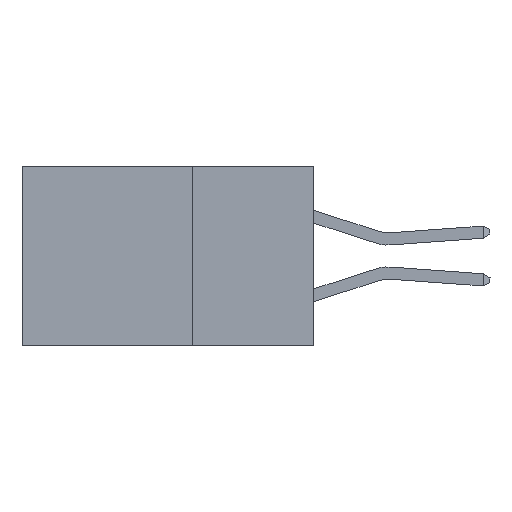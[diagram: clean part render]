
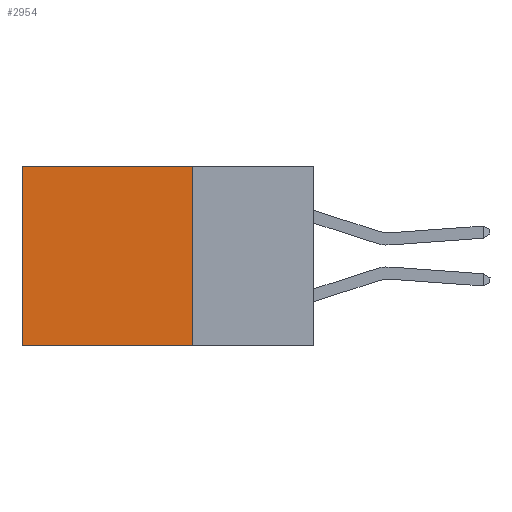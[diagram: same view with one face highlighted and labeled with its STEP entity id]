
A CAD part, left-side view. The second image highlights one B-rep face of the part: STEP entity #2954.
In plain terms, the highlighted planar face has unit normal (-1, 0, 0).
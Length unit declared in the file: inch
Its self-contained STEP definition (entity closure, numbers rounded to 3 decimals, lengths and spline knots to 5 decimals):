
#363 = CARTESIAN_POINT ( 'NONE',  ( 0.2875, 0.6, 0. ) ) ;
#774 = EDGE_CURVE ( 'NONE', #15094, #14902, #2445, .T. ) ;
#1071 = CARTESIAN_POINT ( 'NONE',  ( 0.2875, 0.25, 0. ) ) ;
#1073 = PLANE ( 'NONE',  #17913 ) ;
#1156 = DIRECTION ( 'NONE',  ( 0., 0., -1. ) ) ;
#1989 = EDGE_CURVE ( 'NONE', #2908, #14902, #17103, .T. ) ;
#2445 = LINE ( 'NONE', #4836, #7777 ) ;
#2598 = CARTESIAN_POINT ( 'NONE',  ( 0.2875, 0.25, 0. ) ) ;
#2908 = VERTEX_POINT ( 'NONE', #7260 ) ;
#2954 = ADVANCED_FACE ( 'NONE', ( #10932 ), #1073, .F. ) ;
#3006 = VECTOR ( 'NONE', #1156, 39.37008 ) ;
#4208 = DIRECTION ( 'NONE',  ( 0., 0., -1. ) ) ;
#4836 = CARTESIAN_POINT ( 'NONE',  ( 0.2875, 0.6, 0. ) ) ;
#6017 = ORIENTED_EDGE ( 'NONE', *, *, #1989, .F. ) ;
#6529 = VECTOR ( 'NONE', #10234, 39.37008 ) ;
#6673 = EDGE_CURVE ( 'NONE', #12420, #15094, #7538, .T. ) ;
#6769 = ORIENTED_EDGE ( 'NONE', *, *, #774, .T. ) ;
#6953 = LINE ( 'NONE', #7032, #3006 ) ;
#7032 = CARTESIAN_POINT ( 'NONE',  ( 0.2875, 0.25, 0. ) ) ;
#7049 = ORIENTED_EDGE ( 'NONE', *, *, #10641, .F. ) ;
#7240 = EDGE_LOOP ( 'NONE', ( #6769, #6017, #7049, #16373 ) ) ;
#7260 = CARTESIAN_POINT ( 'NONE',  ( 0.2875, 0.25, -0.37 ) ) ;
#7302 = VECTOR ( 'NONE', #19250, 39.37008 ) ;
#7538 = LINE ( 'NONE', #1071, #7302 ) ;
#7777 = VECTOR ( 'NONE', #10533, 39.37008 ) ;
#9877 = CARTESIAN_POINT ( 'NONE',  ( 0.2875, 0.25, 0. ) ) ;
#10234 = DIRECTION ( 'NONE',  ( 0., 1., 0. ) ) ;
#10533 = DIRECTION ( 'NONE',  ( 0., 0., -1. ) ) ;
#10641 = EDGE_CURVE ( 'NONE', #12420, #2908, #6953, .T. ) ;
#10932 = FACE_OUTER_BOUND ( 'NONE', #7240, .T. ) ;
#12420 = VERTEX_POINT ( 'NONE', #9877 ) ;
#13080 = DIRECTION ( 'NONE',  ( 1., 0., 0. ) ) ;
#14294 = CARTESIAN_POINT ( 'NONE',  ( 0.2875, 0.6, -0.37 ) ) ;
#14902 = VERTEX_POINT ( 'NONE', #14294 ) ;
#15094 = VERTEX_POINT ( 'NONE', #363 ) ;
#16373 = ORIENTED_EDGE ( 'NONE', *, *, #6673, .T. ) ;
#17103 = LINE ( 'NONE', #17872, #6529 ) ;
#17872 = CARTESIAN_POINT ( 'NONE',  ( 0.2875, 0.25, -0.37 ) ) ;
#17913 = AXIS2_PLACEMENT_3D ( 'NONE', #2598, #13080, #4208 ) ;
#19250 = DIRECTION ( 'NONE',  ( 0., 1., 0. ) ) ;
